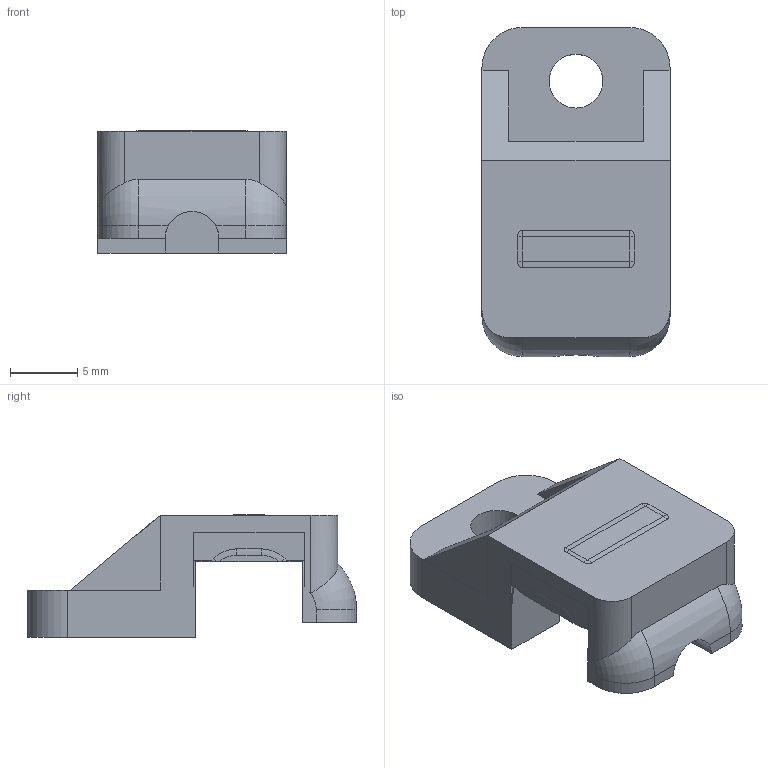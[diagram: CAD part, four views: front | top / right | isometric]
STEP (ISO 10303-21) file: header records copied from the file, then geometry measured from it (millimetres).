
FILE_DESCRIPTION (( 'STEP AP203' ), '1' );
FILE_NAME ('WTF-9_hillbilly_mag_catch_mount.STEP', '2020-05-09T08:58:17', ( '' ), ( '' ), 'SwSTEP 2.0', 'SolidWorks 2016', '' );
FILE_SCHEMA (( 'CONFIG_CONTROL_DESIGN' ));
Length unit declared in the file: millimetre
Products named in the file (2): WTF HILLBILLY FINAL_12; WTF-9_hillbilly_mag_catch_mount
Assembly tree (1 placements, depth 2):
  WTF-9_hillbilly_mag_catch_mount
    WTF HILLBILLY FINAL_12
Bounding box: 14 x 24.5 x 9.1 mm (x, y, z)
Volume: 1503.1 mm3; surface area: 1478.5 mm2
Topology: 1 solids, 3 shells, 82 faces, 219 edges, 144 vertices
Faces by surface type: plane 46, cylinder 22, torus 12, bspline 2
Full cylindrical faces by diameter (mm): 4 x1
Entity records: 3775 total; most frequent: CARTESIAN_POINT 1614, ORIENTED_EDGE 436, DIRECTION 388, EDGE_CURVE 218, VERTEX_POINT 144, AXIS2_PLACEMENT_3D 133, VECTOR 122, LINE 122
